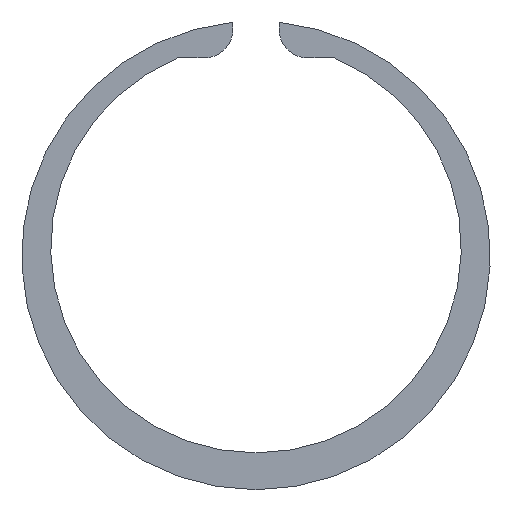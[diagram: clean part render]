
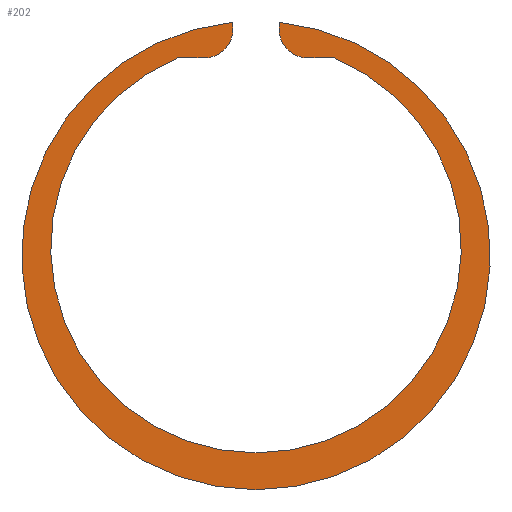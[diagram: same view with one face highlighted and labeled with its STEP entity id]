
A CAD part, front view. The second image highlights one B-rep face of the part: STEP entity #202.
In plain terms, the highlighted planar face has unit normal (0, -1, 0).
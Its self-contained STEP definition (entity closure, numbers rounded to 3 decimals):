
#2 = VERTEX_POINT ( 'NONE', #8 ) ;
#7 = LINE ( 'NONE', #18, #121 ) ;
#8 = CARTESIAN_POINT ( 'NONE',  ( -0.635, -0.198, 6.433 ) ) ;
#11 = DIRECTION ( 'NONE',  ( 0., 0., -1. ) ) ;
#14 = DIRECTION ( 'NONE',  ( 0., 0., -1. ) ) ;
#15 = DIRECTION ( 'NONE',  ( 0., 1., 0. ) ) ;
#16 = CARTESIAN_POINT ( 'NONE',  ( -1.429, -0.198, 6.242 ) ) ;
#18 = CARTESIAN_POINT ( 'NONE',  ( -0.635, -0.198, 6.242 ) ) ;
#20 = AXIS2_PLACEMENT_3D ( 'NONE', #412, #396, #395 ) ;
#22 = VERTEX_POINT ( 'NONE', #402 ) ;
#25 = DIRECTION ( 'NONE',  ( 0., 0., 1. ) ) ;
#30 = DIRECTION ( 'NONE',  ( 0., 0., -1. ) ) ;
#31 = DIRECTION ( 'NONE',  ( 0., 1., 0. ) ) ;
#32 = CARTESIAN_POINT ( 'NONE',  ( 0., -0.198, 0.216 ) ) ;
#33 = DIRECTION ( 'NONE',  ( 1., 0., 0. ) ) ;
#34 = AXIS2_PLACEMENT_3D ( 'NONE', #408, #407, #404 ) ;
#35 = CARTESIAN_POINT ( 'NONE',  ( -2.169, -0.198, 5.448 ) ) ;
#41 = CARTESIAN_POINT ( 'NONE',  ( 1.429, -0.198, 6.242 ) ) ;
#42 = CARTESIAN_POINT ( 'NONE',  ( 1.429, -0.198, 5.448 ) ) ;
#45 = DIRECTION ( 'NONE',  ( 1., 0., 0. ) ) ;
#46 = DIRECTION ( 'NONE',  ( 0., 0., -1. ) ) ;
#49 = DIRECTION ( 'NONE',  ( 0., 1., 0. ) ) ;
#55 = CARTESIAN_POINT ( 'NONE',  ( 0., -0.198, 0. ) ) ;
#58 = DIRECTION ( 'NONE',  ( 0., 0., -1. ) ) ;
#61 = CARTESIAN_POINT ( 'NONE',  ( 0.635, -0.198, 6.242 ) ) ;
#63 = CARTESIAN_POINT ( 'NONE',  ( -2.169, -0.198, 5.448 ) ) ;
#65 = DIRECTION ( 'NONE',  ( 0., 0., -1. ) ) ;
#67 = DIRECTION ( 'NONE',  ( 0., 1., 0. ) ) ;
#69 = CARTESIAN_POINT ( 'NONE',  ( 0., -0.198, 0.216 ) ) ;
#89 = CARTESIAN_POINT ( 'NONE',  ( -0.635, -0.198, 6.242 ) ) ;
#91 = CARTESIAN_POINT ( 'NONE',  ( -1.429, -0.198, 5.448 ) ) ;
#102 = CARTESIAN_POINT ( 'NONE',  ( 0., -0.198, -6.464 ) ) ;
#111 = CARTESIAN_POINT ( 'NONE',  ( 0.635, -0.198, 6.242 ) ) ;
#120 = CARTESIAN_POINT ( 'NONE',  ( 1.429, -0.198, 5.448 ) ) ;
#121 = VECTOR ( 'NONE', #25, 1000. ) ;
#126 = VECTOR ( 'NONE', #33, 1000. ) ;
#127 = CIRCLE ( 'NONE', #290, 0.794 ) ;
#130 = VECTOR ( 'NONE', #45, 1000. ) ;
#132 = LINE ( 'NONE', #35, #126 ) ;
#133 = CIRCLE ( 'NONE', #294, 5.664 ) ;
#134 = VECTOR ( 'NONE', #58, 1000. ) ;
#138 = LINE ( 'NONE', #42, #130 ) ;
#139 = LINE ( 'NONE', #61, #134 ) ;
#144 = CARTESIAN_POINT ( 'NONE',  ( 2.169, -0.198, 5.448 ) ) ;
#147 = CIRCLE ( 'NONE', #297, 6.464 ) ;
#149 = CIRCLE ( 'NONE', #296, 0.794 ) ;
#153 = CIRCLE ( 'NONE', #305, 5.664 ) ;
#166 = EDGE_CURVE ( 'NONE', #252, #2, #187, .T. ) ;
#181 = DIRECTION ( 'NONE',  ( 0., -1., 0. ) ) ;
#187 = CIRCLE ( 'NONE', #34, 6.464 ) ;
#198 = FACE_OUTER_BOUND ( 'NONE', #378, .T. ) ;
#202 = ADVANCED_FACE ( 'NONE', ( #198 ), #397, .T. ) ;
#233 = ORIENTED_EDGE ( 'NONE', *, *, #321, .F. ) ;
#234 = ORIENTED_EDGE ( 'NONE', *, *, #323, .T. ) ;
#235 = ORIENTED_EDGE ( 'NONE', *, *, #324, .T. ) ;
#241 = ORIENTED_EDGE ( 'NONE', *, *, #329, .T. ) ;
#242 = ORIENTED_EDGE ( 'NONE', *, *, #314, .T. ) ;
#244 = ORIENTED_EDGE ( 'NONE', *, *, #330, .T. ) ;
#245 = ORIENTED_EDGE ( 'NONE', *, *, #333, .T. ) ;
#246 = ORIENTED_EDGE ( 'NONE', *, *, #335, .F. ) ;
#247 = ORIENTED_EDGE ( 'NONE', *, *, #337, .T. ) ;
#248 = ORIENTED_EDGE ( 'NONE', *, *, #166, .F. ) ;
#252 = VERTEX_POINT ( 'NONE', #102 ) ;
#290 = AXIS2_PLACEMENT_3D ( 'NONE', #16, #15, #14 ) ;
#294 = AXIS2_PLACEMENT_3D ( 'NONE', #32, #31, #30 ) ;
#296 = AXIS2_PLACEMENT_3D ( 'NONE', #41, #181, #11 ) ;
#297 = AXIS2_PLACEMENT_3D ( 'NONE', #55, #49, #46 ) ;
#305 = AXIS2_PLACEMENT_3D ( 'NONE', #69, #67, #65 ) ;
#314 = EDGE_CURVE ( 'NONE', #387, #359, #153, .T. ) ;
#321 = EDGE_CURVE ( 'NONE', #22, #252, #147, .T. ) ;
#323 = EDGE_CURVE ( 'NONE', #22, #381, #139, .T. ) ;
#324 = EDGE_CURVE ( 'NONE', #381, #386, #149, .T. ) ;
#329 = EDGE_CURVE ( 'NONE', #386, #387, #138, .T. ) ;
#330 = EDGE_CURVE ( 'NONE', #359, #409, #133, .T. ) ;
#333 = EDGE_CURVE ( 'NONE', #409, #393, #132, .T. ) ;
#335 = EDGE_CURVE ( 'NONE', #400, #393, #127, .T. ) ;
#337 = EDGE_CURVE ( 'NONE', #400, #2, #7, .T. ) ;
#359 = VERTEX_POINT ( 'NONE', #405 ) ;
#378 = EDGE_LOOP ( 'NONE', ( #233, #234, #235, #241, #242, #244, #245, #246, #247, #248 ) ) ;
#381 = VERTEX_POINT ( 'NONE', #111 ) ;
#386 = VERTEX_POINT ( 'NONE', #120 ) ;
#387 = VERTEX_POINT ( 'NONE', #144 ) ;
#393 = VERTEX_POINT ( 'NONE', #91 ) ;
#395 = DIRECTION ( 'NONE',  ( 0., 0., -1. ) ) ;
#396 = DIRECTION ( 'NONE',  ( 0., -1., 0. ) ) ;
#397 = PLANE ( 'NONE',  #20 ) ;
#400 = VERTEX_POINT ( 'NONE', #89 ) ;
#402 = CARTESIAN_POINT ( 'NONE',  ( 0.635, -0.198, 6.433 ) ) ;
#404 = DIRECTION ( 'NONE',  ( 0., 0., -1. ) ) ;
#405 = CARTESIAN_POINT ( 'NONE',  ( 0., -0.198, -5.448 ) ) ;
#407 = DIRECTION ( 'NONE',  ( 0., 1., 0. ) ) ;
#408 = CARTESIAN_POINT ( 'NONE',  ( 0., -0.198, 0. ) ) ;
#409 = VERTEX_POINT ( 'NONE', #63 ) ;
#412 = CARTESIAN_POINT ( 'NONE',  ( 1.429, -0.198, 6.242 ) ) ;
